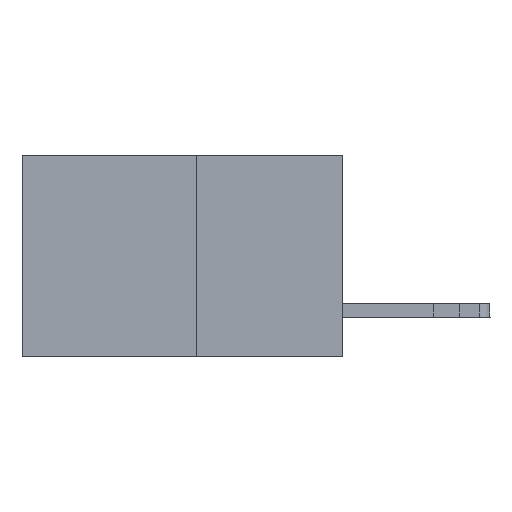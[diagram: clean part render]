
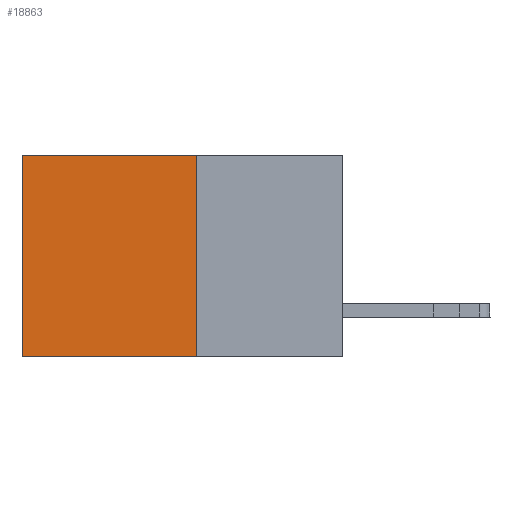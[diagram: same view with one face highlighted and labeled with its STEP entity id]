
A CAD part, left-side view. The second image highlights one B-rep face of the part: STEP entity #18863.
In plain terms, the highlighted planar face has unit normal (-1, 0, 0).
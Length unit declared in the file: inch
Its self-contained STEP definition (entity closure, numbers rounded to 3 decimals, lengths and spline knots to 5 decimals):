
#731 = EDGE_CURVE ( 'NONE', #18713, #16889, #16716, .T. ) ;
#1878 = VECTOR ( 'NONE', #6022, 39.37008 ) ;
#2350 = CARTESIAN_POINT ( 'NONE',  ( 0.277, 0.27, 0. ) ) ;
#2602 = DIRECTION ( 'NONE',  ( 1., 0., 0. ) ) ;
#2824 = FACE_OUTER_BOUND ( 'NONE', #18284, .T. ) ;
#3025 = VERTEX_POINT ( 'NONE', #7636 ) ;
#3093 = CARTESIAN_POINT ( 'NONE',  ( 0.277, 0.27, -0.37 ) ) ;
#3234 = DIRECTION ( 'NONE',  ( 0., 0., -1. ) ) ;
#3329 = DIRECTION ( 'NONE',  ( 0., 1., 0. ) ) ;
#5774 = ORIENTED_EDGE ( 'NONE', *, *, #12542, .T. ) ;
#6022 = DIRECTION ( 'NONE',  ( 0., 1., 0. ) ) ;
#6031 = LINE ( 'NONE', #7775, #18315 ) ;
#6311 = CARTESIAN_POINT ( 'NONE',  ( 0.277, 0.27, 0. ) ) ;
#6341 = ORIENTED_EDGE ( 'NONE', *, *, #17218, .T. ) ;
#7579 = LINE ( 'NONE', #6311, #1878 ) ;
#7636 = CARTESIAN_POINT ( 'NONE',  ( 0.277, 0.59, 0. ) ) ;
#7775 = CARTESIAN_POINT ( 'NONE',  ( 0.277, 0.59, -0.37 ) ) ;
#7860 = DIRECTION ( 'NONE',  ( 0., 0., -1. ) ) ;
#8756 = PLANE ( 'NONE',  #14672 ) ;
#10819 = EDGE_CURVE ( 'NONE', #16889, #14870, #14805, .T. ) ;
#12542 = EDGE_CURVE ( 'NONE', #3025, #14870, #6031, .T. ) ;
#13600 = ORIENTED_EDGE ( 'NONE', *, *, #10819, .F. ) ;
#14543 = VECTOR ( 'NONE', #3329, 39.37008 ) ;
#14672 = AXIS2_PLACEMENT_3D ( 'NONE', #17990, #2602, #14788 ) ;
#14788 = DIRECTION ( 'NONE',  ( 0., 0., -1. ) ) ;
#14805 = LINE ( 'NONE', #16669, #14543 ) ;
#14870 = VERTEX_POINT ( 'NONE', #17901 ) ;
#14875 = ORIENTED_EDGE ( 'NONE', *, *, #731, .F. ) ;
#16669 = CARTESIAN_POINT ( 'NONE',  ( 0.277, 0.27, -0.37 ) ) ;
#16716 = LINE ( 'NONE', #3093, #17871 ) ;
#16889 = VERTEX_POINT ( 'NONE', #17054 ) ;
#17054 = CARTESIAN_POINT ( 'NONE',  ( 0.277, 0.27, -0.37 ) ) ;
#17218 = EDGE_CURVE ( 'NONE', #18713, #3025, #7579, .T. ) ;
#17871 = VECTOR ( 'NONE', #7860, 39.37008 ) ;
#17901 = CARTESIAN_POINT ( 'NONE',  ( 0.277, 0.59, -0.37 ) ) ;
#17990 = CARTESIAN_POINT ( 'NONE',  ( 0.277, 0.27, -0.37 ) ) ;
#18284 = EDGE_LOOP ( 'NONE', ( #5774, #13600, #14875, #6341 ) ) ;
#18315 = VECTOR ( 'NONE', #3234, 39.37008 ) ;
#18713 = VERTEX_POINT ( 'NONE', #2350 ) ;
#18863 = ADVANCED_FACE ( 'NONE', ( #2824 ), #8756, .F. ) ;
